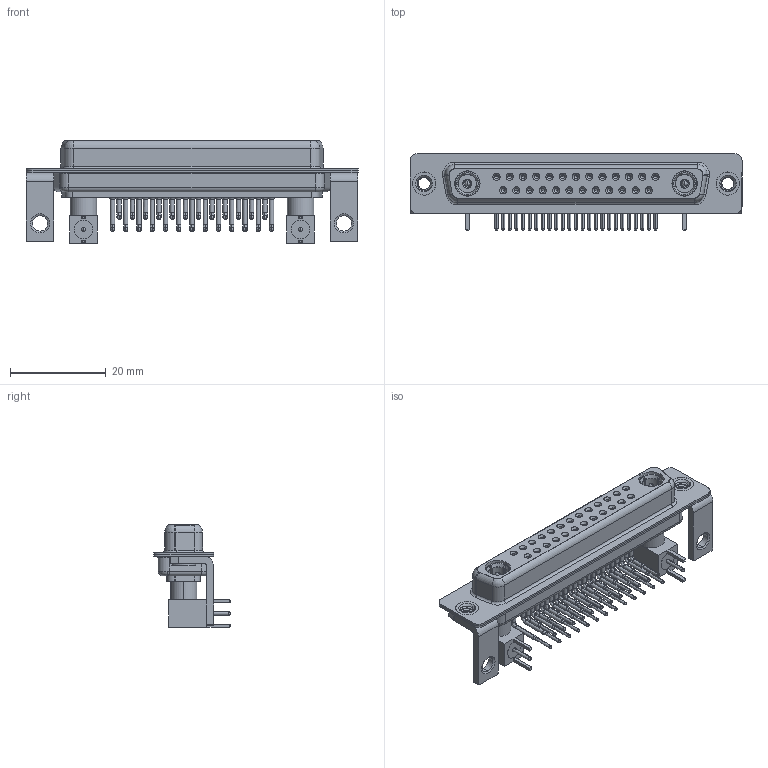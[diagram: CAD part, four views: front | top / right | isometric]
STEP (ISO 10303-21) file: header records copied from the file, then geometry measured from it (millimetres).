
FILE_DESCRIPTION (( 'STEP AP203' ), '1' );
FILE_NAME ('630-27W2640-7TC.STEP', '2022-06-07T18:40:08', ( '' ), ( '' ), 'SwSTEP 2.0', 'SolidWorks 2020', '' );
FILE_SCHEMA (( 'CONFIG_CONTROL_DESIGN' ));
Length unit declared in the file: millimetre
Products named in the file (16): 630Combo Shell Rear_37 Contacts; 630-27W2640-7TC; Co-Ax Plug Assy_RA; Pin_RA; Locking Collar; 630Combo Threaded Rivet_B; 630Combo Contact Row 2; Co-Ax Plug_RA PC Tail; Insulator RA Pin; 630Combo Contact Row 1; RA Back Shell; 630Combo Housing_27W2; Insulator Pin_Straight PC Tail; 630Combo Stabilizer Bracket; 630Combo Shell Front_37 Contacts
Assembly tree (46 placements, depth 3):
  630-27W2640-7TC
    630Combo Housing_27W2
    630Combo Shell Front_37 Contacts
    630Combo Shell Rear_37 Contacts
    630Combo Threaded Rivet_B  x2
    630Combo Stabilizer Bracket  x2
    Co-Ax Plug Assy_RA
      Co-Ax Plug_RA PC Tail
      Insulator Pin_Straight PC Tail
      Pin_RA
      Locking Collar
      RA Back Shell
      Insulator RA Pin
    Co-Ax Plug Assy_RA
      Co-Ax Plug_RA PC Tail
      Insulator Pin_Straight PC Tail
      Pin_RA
      Locking Collar
      RA Back Shell
      Insulator RA Pin
    630Combo Contact Row 1  x13
    630Combo Contact Row 2  x12
Bounding box: 69.4 x 16 x 21.41 mm (x, y, z)
Volume: 6268.1 mm3; surface area: 14382.2 mm2
Topology: 44 solids, 44 shells, 1978 faces, 4962 edges, 3120 vertices
Faces by surface type: cylinder 860, plane 596, cone 337, bspline 108, torus 69, sphere 8
Entity records: 28888 total; most frequent: CARTESIAN_POINT 6115, DIRECTION 4659, ORIENTED_EDGE 3922, EDGE_CURVE 1961, AXIS2_PLACEMENT_3D 1927, VERTEX_POINT 1249, CIRCLE 1045, EDGE_LOOP 1028
